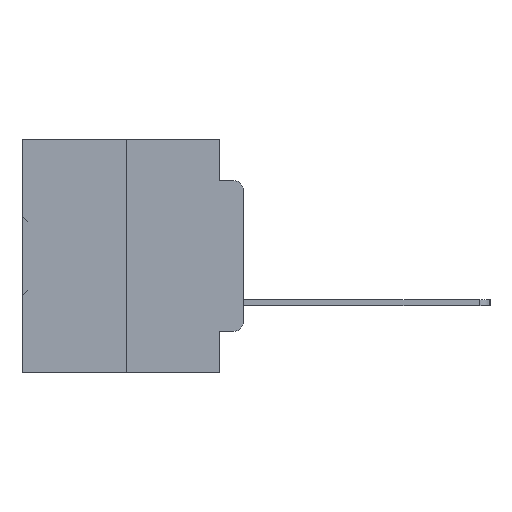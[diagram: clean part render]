
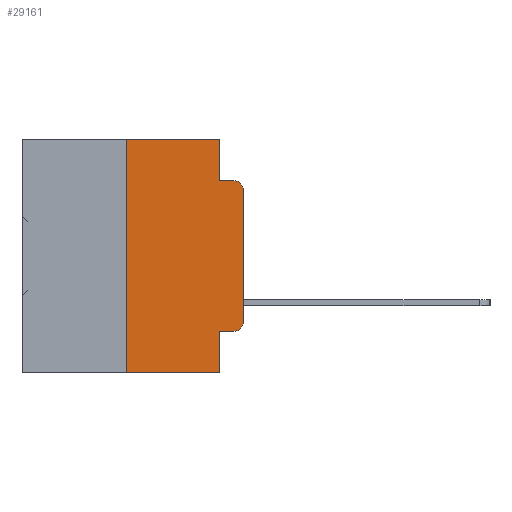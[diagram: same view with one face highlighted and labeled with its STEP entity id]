
A CAD part, left-side view. The second image highlights one B-rep face of the part: STEP entity #29161.
In plain terms, the highlighted planar face has unit normal (-1, 0, 0).
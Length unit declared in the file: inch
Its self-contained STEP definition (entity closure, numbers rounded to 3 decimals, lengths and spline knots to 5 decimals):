
#1470 = LINE ( 'NONE', #9643, #31150 ) ;
#1537 = EDGE_CURVE ( 'NONE', #12071, #14517, #14066, .T. ) ;
#1988 = VERTEX_POINT ( 'NONE', #28917 ) ;
#2516 = CARTESIAN_POINT ( 'NONE',  ( 0., 0.473, 0. ) ) ;
#3446 = ORIENTED_EDGE ( 'NONE', *, *, #7405, .F. ) ;
#3772 = EDGE_CURVE ( 'NONE', #14517, #30224, #27786, .T. ) ;
#3920 = LINE ( 'NONE', #25267, #19329 ) ;
#4316 = ORIENTED_EDGE ( 'NONE', *, *, #11329, .T. ) ;
#4648 = CARTESIAN_POINT ( 'NONE',  ( 0., 0.051, 0. ) ) ;
#4813 = VECTOR ( 'NONE', #11426, 39.37008 ) ;
#4848 = VECTOR ( 'NONE', #17654, 39.37008 ) ;
#5297 = ORIENTED_EDGE ( 'NONE', *, *, #33074, .T. ) ;
#5437 = DIRECTION ( 'NONE',  ( 0., 0., -1. ) ) ;
#6139 = ORIENTED_EDGE ( 'NONE', *, *, #9375, .F. ) ;
#6370 = VERTEX_POINT ( 'NONE', #31191 ) ;
#7011 = CARTESIAN_POINT ( 'NONE',  ( 0., 0.25, 0. ) ) ;
#7071 = CARTESIAN_POINT ( 'NONE',  ( 0., 0.02, -0.3915 ) ) ;
#7279 = DIRECTION ( 'NONE',  ( 0., 0., 1. ) ) ;
#7379 = VERTEX_POINT ( 'NONE', #18980 ) ;
#7405 = EDGE_CURVE ( 'NONE', #30224, #15028, #33079, .T. ) ;
#7550 = VERTEX_POINT ( 'NONE', #11160 ) ;
#7584 = ORIENTED_EDGE ( 'NONE', *, *, #9880, .T. ) ;
#9158 = CIRCLE ( 'NONE', #12839, 0.02 ) ;
#9354 = ORIENTED_EDGE ( 'NONE', *, *, #20973, .T. ) ;
#9375 = EDGE_CURVE ( 'NONE', #15028, #7379, #26700, .T. ) ;
#9425 = ORIENTED_EDGE ( 'NONE', *, *, #34967, .F. ) ;
#9643 = CARTESIAN_POINT ( 'NONE',  ( 0., 0.473, -0.5 ) ) ;
#9880 = EDGE_CURVE ( 'NONE', #12071, #1988, #1470, .T. ) ;
#9954 = LINE ( 'NONE', #22743, #30938 ) ;
#10035 = DIRECTION ( 'NONE',  ( 0., 0., -1. ) ) ;
#11022 = DIRECTION ( 'NONE',  ( 0., 0., 1. ) ) ;
#11160 = CARTESIAN_POINT ( 'NONE',  ( 0., 0.02, -0.4115 ) ) ;
#11329 = EDGE_CURVE ( 'NONE', #24193, #7379, #35073, .T. ) ;
#11426 = DIRECTION ( 'NONE',  ( 0., 0., -1. ) ) ;
#11677 = ORIENTED_EDGE ( 'NONE', *, *, #3772, .F. ) ;
#12071 = VERTEX_POINT ( 'NONE', #32895 ) ;
#12372 = CARTESIAN_POINT ( 'NONE',  ( 0., 0.25, 0. ) ) ;
#12839 = AXIS2_PLACEMENT_3D ( 'NONE', #7071, #27154, #10035 ) ;
#14066 = LINE ( 'NONE', #12372, #28350 ) ;
#14088 = PLANE ( 'NONE',  #14097 ) ;
#14097 = AXIS2_PLACEMENT_3D ( 'NONE', #2516, #22755, #5437 ) ;
#14316 = CARTESIAN_POINT ( 'NONE',  ( 0., 0.051, 0. ) ) ;
#14517 = VERTEX_POINT ( 'NONE', #7011 ) ;
#14856 = ORIENTED_EDGE ( 'NONE', *, *, #25450, .T. ) ;
#15028 = VERTEX_POINT ( 'NONE', #29300 ) ;
#15434 = DIRECTION ( 'NONE',  ( 0., -1., 0. ) ) ;
#15945 = CARTESIAN_POINT ( 'NONE',  ( 0., 0., -0.3915 ) ) ;
#16091 = DIRECTION ( 'NONE',  ( 0., -1., 0. ) ) ;
#16985 = DIRECTION ( 'NONE',  ( -1., 0., 0. ) ) ;
#17439 = CARTESIAN_POINT ( 'NONE',  ( 0., 0.473, 0. ) ) ;
#17654 = DIRECTION ( 'NONE',  ( 0., -1., 0. ) ) ;
#18820 = CARTESIAN_POINT ( 'NONE',  ( 0., 0., -0.1085 ) ) ;
#18980 = CARTESIAN_POINT ( 'NONE',  ( 0., 0.02, -0.0885 ) ) ;
#19003 = CARTESIAN_POINT ( 'NONE',  ( 0., 0.051, -0.0885 ) ) ;
#19329 = VECTOR ( 'NONE', #11022, 39.37008 ) ;
#19936 = VERTEX_POINT ( 'NONE', #15945 ) ;
#20054 = VECTOR ( 'NONE', #16091, 39.37008 ) ;
#20973 = EDGE_CURVE ( 'NONE', #19936, #24193, #3920, .T. ) ;
#22743 = CARTESIAN_POINT ( 'NONE',  ( 0., 0.051, -0.4115 ) ) ;
#22755 = DIRECTION ( 'NONE',  ( 1., 0., 0. ) ) ;
#24193 = VERTEX_POINT ( 'NONE', #18820 ) ;
#24805 = DIRECTION ( 'NONE',  ( 0., 0., -1. ) ) ;
#25267 = CARTESIAN_POINT ( 'NONE',  ( 0., 0., 0. ) ) ;
#25418 = AXIS2_PLACEMENT_3D ( 'NONE', #34020, #16985, #36834 ) ;
#25450 = EDGE_CURVE ( 'NONE', #7550, #19936, #9158, .T. ) ;
#25508 = VECTOR ( 'NONE', #24805, 39.37008 ) ;
#26392 = FACE_OUTER_BOUND ( 'NONE', #29580, .T. ) ;
#26700 = LINE ( 'NONE', #19003, #20054 ) ;
#26862 = LINE ( 'NONE', #14316, #4813 ) ;
#27154 = DIRECTION ( 'NONE',  ( -1., 0., 0. ) ) ;
#27786 = LINE ( 'NONE', #17439, #4848 ) ;
#28350 = VECTOR ( 'NONE', #7279, 39.37008 ) ;
#28917 = CARTESIAN_POINT ( 'NONE',  ( 0., 0.051, -0.5 ) ) ;
#29161 = ADVANCED_FACE ( 'NONE', ( #26392 ), #14088, .F. ) ;
#29300 = CARTESIAN_POINT ( 'NONE',  ( 0., 0.051, -0.0885 ) ) ;
#29580 = EDGE_LOOP ( 'NONE', ( #9354, #4316, #6139, #3446, #11677, #34432, #7584, #9425, #5297, #14856 ) ) ;
#30224 = VERTEX_POINT ( 'NONE', #30315 ) ;
#30315 = CARTESIAN_POINT ( 'NONE',  ( 0., 0.051, 0. ) ) ;
#30938 = VECTOR ( 'NONE', #31139, 39.37008 ) ;
#31139 = DIRECTION ( 'NONE',  ( 0., -1., 0. ) ) ;
#31150 = VECTOR ( 'NONE', #15434, 39.37008 ) ;
#31191 = CARTESIAN_POINT ( 'NONE',  ( 0., 0.051, -0.4115 ) ) ;
#32895 = CARTESIAN_POINT ( 'NONE',  ( 0., 0.25, -0.5 ) ) ;
#33074 = EDGE_CURVE ( 'NONE', #6370, #7550, #9954, .T. ) ;
#33079 = LINE ( 'NONE', #4648, #25508 ) ;
#34020 = CARTESIAN_POINT ( 'NONE',  ( 0., 0.02, -0.1085 ) ) ;
#34432 = ORIENTED_EDGE ( 'NONE', *, *, #1537, .F. ) ;
#34967 = EDGE_CURVE ( 'NONE', #6370, #1988, #26862, .T. ) ;
#35073 = CIRCLE ( 'NONE', #25418, 0.02 ) ;
#36834 = DIRECTION ( 'NONE',  ( 0., 0., -1. ) ) ;
